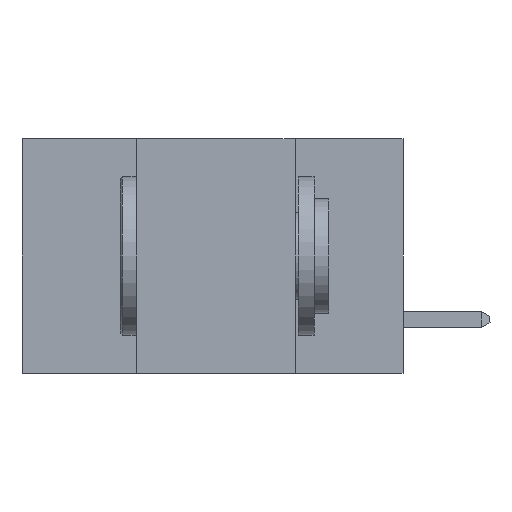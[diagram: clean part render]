
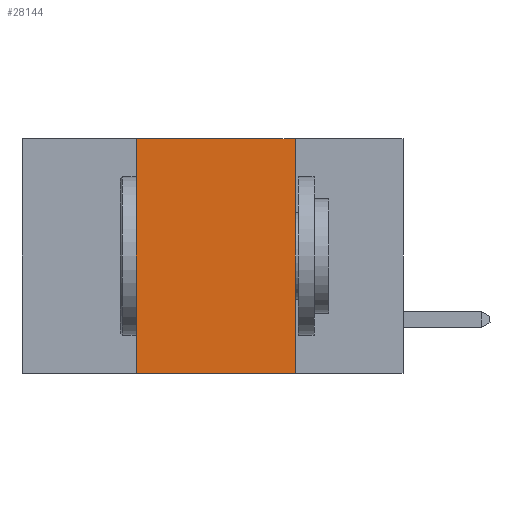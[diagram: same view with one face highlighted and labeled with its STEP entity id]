
A CAD part, left-side view. The second image highlights one B-rep face of the part: STEP entity #28144.
In plain terms, the highlighted planar face has unit normal (-1, 0, 0).
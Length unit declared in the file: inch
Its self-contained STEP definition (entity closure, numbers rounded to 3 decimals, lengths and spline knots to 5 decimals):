
#1089 = DIRECTION ( 'NONE',  ( 0., 0., -1. ) ) ;
#1170 = VECTOR ( 'NONE', #15568, 39.37008 ) ;
#1563 = EDGE_CURVE ( 'NONE', #7247, #16402, #20557, .T. ) ;
#1688 = CARTESIAN_POINT ( 'NONE',  ( 0., 0.17, -0.37 ) ) ;
#2735 = ORIENTED_EDGE ( 'NONE', *, *, #6728, .F. ) ;
#3582 = CARTESIAN_POINT ( 'NONE',  ( 0., 0.42, 0. ) ) ;
#4377 = LINE ( 'NONE', #26733, #5167 ) ;
#5167 = VECTOR ( 'NONE', #21803, 39.37008 ) ;
#6728 = EDGE_CURVE ( 'NONE', #30690, #19993, #4377, .T. ) ;
#7085 = VECTOR ( 'NONE', #18778, 39.37008 ) ;
#7247 = VERTEX_POINT ( 'NONE', #11038 ) ;
#8360 = EDGE_LOOP ( 'NONE', ( #22075, #2735, #14370, #15960 ) ) ;
#11038 = CARTESIAN_POINT ( 'NONE',  ( 0., 0.42, -0.37 ) ) ;
#12363 = EDGE_CURVE ( 'NONE', #7247, #30690, #16288, .T. ) ;
#14370 = ORIENTED_EDGE ( 'NONE', *, *, #12363, .F. ) ;
#15568 = DIRECTION ( 'NONE',  ( 0., 0., -1. ) ) ;
#15960 = ORIENTED_EDGE ( 'NONE', *, *, #1563, .T. ) ;
#16288 = LINE ( 'NONE', #3582, #7085 ) ;
#16402 = VERTEX_POINT ( 'NONE', #1688 ) ;
#16405 = DIRECTION ( 'NONE',  ( 1., 0., 0. ) ) ;
#18778 = DIRECTION ( 'NONE',  ( 0., 0., 1. ) ) ;
#19993 = VERTEX_POINT ( 'NONE', #28270 ) ;
#20557 = LINE ( 'NONE', #22922, #27066 ) ;
#21138 = EDGE_CURVE ( 'NONE', #19993, #16402, #27866, .T. ) ;
#21458 = CARTESIAN_POINT ( 'NONE',  ( 0., 0.42, 0. ) ) ;
#21803 = DIRECTION ( 'NONE',  ( 0., -1., 0. ) ) ;
#22075 = ORIENTED_EDGE ( 'NONE', *, *, #21138, .F. ) ;
#22922 = CARTESIAN_POINT ( 'NONE',  ( 0., 0.6, -0.37 ) ) ;
#23016 = FACE_OUTER_BOUND ( 'NONE', #8360, .T. ) ;
#23080 = DIRECTION ( 'NONE',  ( 0., -1., 0. ) ) ;
#25341 = CARTESIAN_POINT ( 'NONE',  ( 0., 0.17, 0. ) ) ;
#26158 = CARTESIAN_POINT ( 'NONE',  ( 0., 0.6, 0. ) ) ;
#26733 = CARTESIAN_POINT ( 'NONE',  ( 0., 0.6, 0. ) ) ;
#27066 = VECTOR ( 'NONE', #23080, 39.37008 ) ;
#27866 = LINE ( 'NONE', #25341, #1170 ) ;
#28144 = ADVANCED_FACE ( 'NONE', ( #23016 ), #31046, .F. ) ;
#28270 = CARTESIAN_POINT ( 'NONE',  ( 0., 0.17, 0. ) ) ;
#30528 = AXIS2_PLACEMENT_3D ( 'NONE', #26158, #16405, #1089 ) ;
#30690 = VERTEX_POINT ( 'NONE', #21458 ) ;
#31046 = PLANE ( 'NONE',  #30528 ) ;
